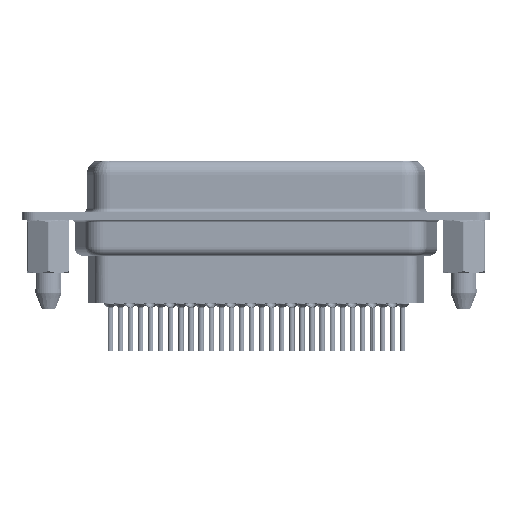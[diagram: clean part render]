
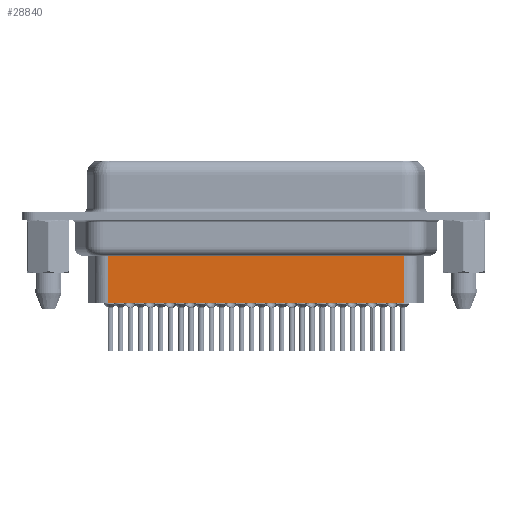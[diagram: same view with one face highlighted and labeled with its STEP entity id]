
A CAD part, front view. The second image highlights one B-rep face of the part: STEP entity #28840.
In plain terms, the highlighted planar face has unit normal (0, -1, 0).
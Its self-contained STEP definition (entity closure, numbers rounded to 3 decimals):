
#285 = CARTESIAN_POINT ( 'NONE',  ( 6.701, -3.5, -4.097 ) ) ;
#2709 = VERTEX_POINT ( 'NONE', #10596 ) ;
#3423 = EDGE_CURVE ( 'NONE', #15410, #6863, #28122, .T. ) ;
#5804 = LINE ( 'NONE', #37764, #18240 ) ;
#6863 = VERTEX_POINT ( 'NONE', #23233 ) ;
#10037 = EDGE_CURVE ( 'NONE', #6863, #2709, #15689, .T. ) ;
#10596 = CARTESIAN_POINT ( 'NONE',  ( 6.701, -3.5, -9.85 ) ) ;
#10867 = VECTOR ( 'NONE', #40749, 1000. ) ;
#11895 = LINE ( 'NONE', #37200, #35211 ) ;
#12048 = FACE_OUTER_BOUND ( 'NONE', #15307, .T. ) ;
#12961 = CARTESIAN_POINT ( 'NONE',  ( 40.339, -3.5, -3.1 ) ) ;
#13854 = ORIENTED_EDGE ( 'NONE', *, *, #10037, .F. ) ;
#15307 = EDGE_LOOP ( 'NONE', ( #22375, #28231, #26740, #13854 ) ) ;
#15410 = VERTEX_POINT ( 'NONE', #30306 ) ;
#15689 = LINE ( 'NONE', #21937, #30846 ) ;
#18240 = VECTOR ( 'NONE', #34454, 1000. ) ;
#18297 = DIRECTION ( 'NONE',  ( 0., 0., -1. ) ) ;
#21562 = DIRECTION ( 'NONE',  ( 0., -1., 0. ) ) ;
#21937 = CARTESIAN_POINT ( 'NONE',  ( 6.701, -3.5, -9.85 ) ) ;
#22375 = ORIENTED_EDGE ( 'NONE', *, *, #3423, .F. ) ;
#23233 = CARTESIAN_POINT ( 'NONE',  ( 40.339, -3.5, -9.85 ) ) ;
#23721 = EDGE_CURVE ( 'NONE', #15410, #24599, #5804, .T. ) ;
#24475 = AXIS2_PLACEMENT_3D ( 'NONE', #28232, #21562, #40860 ) ;
#24599 = VERTEX_POINT ( 'NONE', #285 ) ;
#26740 = ORIENTED_EDGE ( 'NONE', *, *, #30765, .T. ) ;
#28122 = LINE ( 'NONE', #12961, #10867 ) ;
#28231 = ORIENTED_EDGE ( 'NONE', *, *, #23721, .T. ) ;
#28232 = CARTESIAN_POINT ( 'NONE',  ( 6.701, -3.5, -3.1 ) ) ;
#28840 = ADVANCED_FACE ( 'NONE', ( #12048 ), #34049, .T. ) ;
#30306 = CARTESIAN_POINT ( 'NONE',  ( 40.339, -3.5, -4.097 ) ) ;
#30765 = EDGE_CURVE ( 'NONE', #24599, #2709, #11895, .T. ) ;
#30846 = VECTOR ( 'NONE', #34617, 1000. ) ;
#34049 = PLANE ( 'NONE',  #24475 ) ;
#34454 = DIRECTION ( 'NONE',  ( -1., 0., 0. ) ) ;
#34617 = DIRECTION ( 'NONE',  ( -1., 0., 0. ) ) ;
#35211 = VECTOR ( 'NONE', #18297, 1000. ) ;
#37200 = CARTESIAN_POINT ( 'NONE',  ( 6.701, -3.5, -3.1 ) ) ;
#37764 = CARTESIAN_POINT ( 'NONE',  ( 6.454, -3.5, -4.097 ) ) ;
#40749 = DIRECTION ( 'NONE',  ( 0., 0., -1. ) ) ;
#40860 = DIRECTION ( 'NONE',  ( 1., 0., 0. ) ) ;
